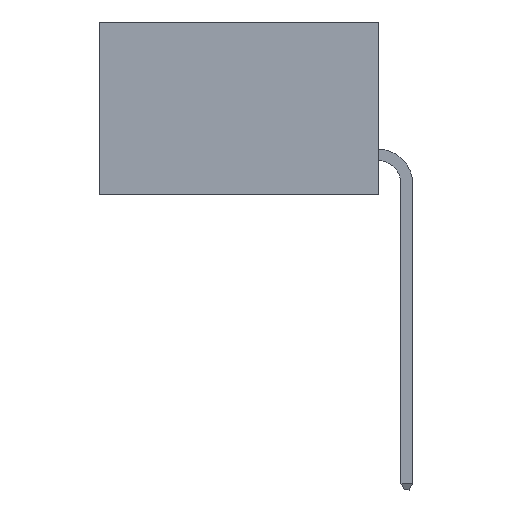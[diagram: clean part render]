
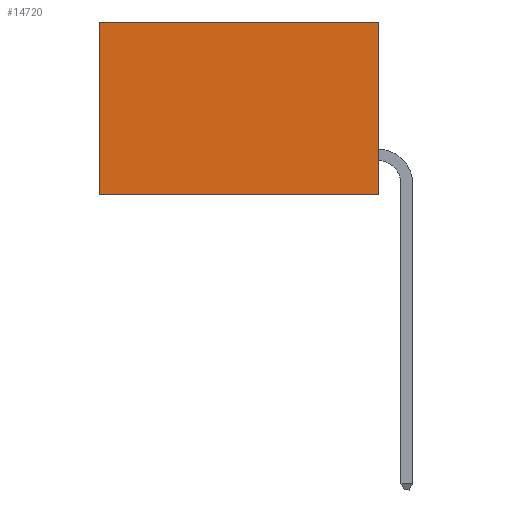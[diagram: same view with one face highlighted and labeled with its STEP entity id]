
A CAD part, left-side view. The second image highlights one B-rep face of the part: STEP entity #14720.
In plain terms, the highlighted planar face has unit normal (-1, 0, 0).
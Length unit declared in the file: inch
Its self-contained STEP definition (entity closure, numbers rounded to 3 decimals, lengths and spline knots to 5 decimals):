
#871 = CARTESIAN_POINT ( 'NONE',  ( 0.2615, 0., -0.37 ) ) ;
#1246 = VERTEX_POINT ( 'NONE', #13106 ) ;
#2254 = VECTOR ( 'NONE', #5730, 39.37008 ) ;
#2370 = CARTESIAN_POINT ( 'NONE',  ( 0.2615, 0., 0. ) ) ;
#2457 = VERTEX_POINT ( 'NONE', #15025 ) ;
#2539 = DIRECTION ( 'NONE',  ( 0., 0., -1. ) ) ;
#2780 = VECTOR ( 'NONE', #2539, 39.37008 ) ;
#3067 = DIRECTION ( 'NONE',  ( 0., 1., 0. ) ) ;
#3365 = CARTESIAN_POINT ( 'NONE',  ( 0.2615, 0.6, -0.37 ) ) ;
#3894 = DIRECTION ( 'NONE',  ( 0., 0., -1. ) ) ;
#3895 = EDGE_CURVE ( 'NONE', #2457, #9633, #7281, .T. ) ;
#5730 = DIRECTION ( 'NONE',  ( 0., 1., 0. ) ) ;
#5911 = ORIENTED_EDGE ( 'NONE', *, *, #10839, .F. ) ;
#6704 = EDGE_CURVE ( 'NONE', #1246, #16807, #9994, .T. ) ;
#6916 = VECTOR ( 'NONE', #3067, 39.37008 ) ;
#7281 = LINE ( 'NONE', #2370, #2254 ) ;
#7341 = LINE ( 'NONE', #871, #8004 ) ;
#8004 = VECTOR ( 'NONE', #3894, 39.37008 ) ;
#9618 = ORIENTED_EDGE ( 'NONE', *, *, #6704, .F. ) ;
#9633 = VERTEX_POINT ( 'NONE', #17894 ) ;
#9994 = LINE ( 'NONE', #20106, #6916 ) ;
#10669 = ORIENTED_EDGE ( 'NONE', *, *, #18223, .T. ) ;
#10839 = EDGE_CURVE ( 'NONE', #2457, #1246, #7341, .T. ) ;
#11109 = DIRECTION ( 'NONE',  ( 1., 0., 0. ) ) ;
#12783 = AXIS2_PLACEMENT_3D ( 'NONE', #17866, #11109, #19539 ) ;
#13106 = CARTESIAN_POINT ( 'NONE',  ( 0.2615, 0., -0.37 ) ) ;
#13364 = ORIENTED_EDGE ( 'NONE', *, *, #3895, .T. ) ;
#14720 = ADVANCED_FACE ( 'NONE', ( #16195 ), #21111, .F. ) ;
#15025 = CARTESIAN_POINT ( 'NONE',  ( 0.2615, 0., 0. ) ) ;
#15984 = CARTESIAN_POINT ( 'NONE',  ( 0.2615, 0.6, -0.37 ) ) ;
#16195 = FACE_OUTER_BOUND ( 'NONE', #16779, .T. ) ;
#16779 = EDGE_LOOP ( 'NONE', ( #10669, #9618, #5911, #13364 ) ) ;
#16807 = VERTEX_POINT ( 'NONE', #3365 ) ;
#17866 = CARTESIAN_POINT ( 'NONE',  ( 0.2615, 0., -0.37 ) ) ;
#17890 = LINE ( 'NONE', #15984, #2780 ) ;
#17894 = CARTESIAN_POINT ( 'NONE',  ( 0.2615, 0.6, 0. ) ) ;
#18223 = EDGE_CURVE ( 'NONE', #9633, #16807, #17890, .T. ) ;
#19539 = DIRECTION ( 'NONE',  ( 0., 0., -1. ) ) ;
#20106 = CARTESIAN_POINT ( 'NONE',  ( 0.2615, 0., -0.37 ) ) ;
#21111 = PLANE ( 'NONE',  #12783 ) ;
